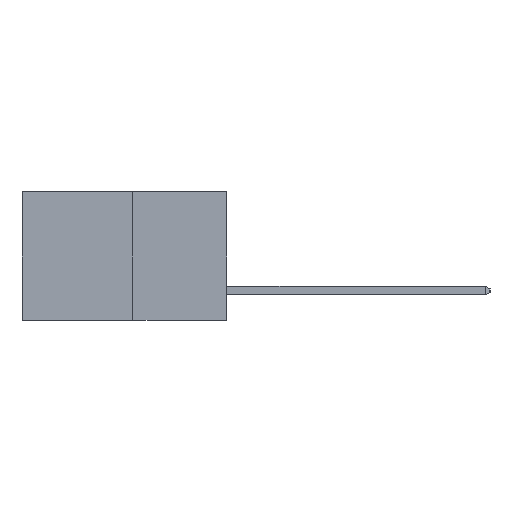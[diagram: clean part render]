
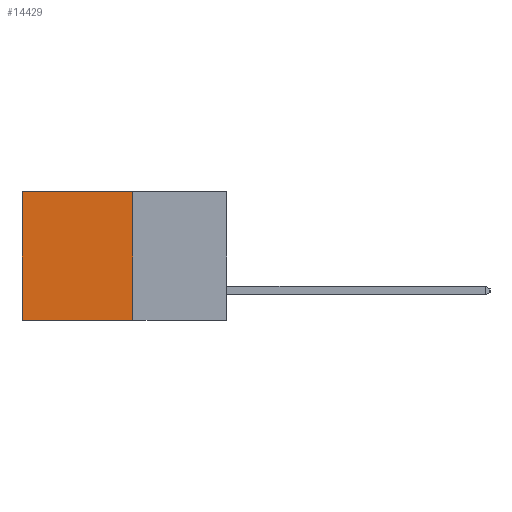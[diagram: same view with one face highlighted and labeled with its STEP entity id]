
A CAD part, left-side view. The second image highlights one B-rep face of the part: STEP entity #14429.
In plain terms, the highlighted planar face has unit normal (-1, 0, 0).
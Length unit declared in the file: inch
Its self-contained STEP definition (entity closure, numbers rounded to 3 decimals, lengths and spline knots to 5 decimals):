
#193 = CARTESIAN_POINT ( 'NONE',  ( 0.277, 0.27, -0.37 ) ) ;
#195 = CARTESIAN_POINT ( 'NONE',  ( 0.277, 0.59, -0.37 ) ) ;
#869 = VECTOR ( 'NONE', #995, 39.37008 ) ;
#995 = DIRECTION ( 'NONE',  ( 0., 0., -1. ) ) ;
#1195 = EDGE_LOOP ( 'NONE', ( #20347, #8211, #4440, #3607 ) ) ;
#1644 = CARTESIAN_POINT ( 'NONE',  ( 0.277, 0.27, -0.37 ) ) ;
#3379 = LINE ( 'NONE', #17132, #8006 ) ;
#3607 = ORIENTED_EDGE ( 'NONE', *, *, #5370, .T. ) ;
#3786 = DIRECTION ( 'NONE',  ( 1., 0., 0. ) ) ;
#4333 = VERTEX_POINT ( 'NONE', #16127 ) ;
#4440 = ORIENTED_EDGE ( 'NONE', *, *, #21651, .F. ) ;
#5370 = EDGE_CURVE ( 'NONE', #9644, #12560, #3379, .T. ) ;
#5723 = EDGE_CURVE ( 'NONE', #12560, #4333, #15222, .T. ) ;
#5804 = DIRECTION ( 'NONE',  ( 0., 0., -1. ) ) ;
#5979 = LINE ( 'NONE', #16025, #10527 ) ;
#6331 = LINE ( 'NONE', #20558, #10337 ) ;
#8006 = VECTOR ( 'NONE', #17205, 39.37008 ) ;
#8211 = ORIENTED_EDGE ( 'NONE', *, *, #9606, .F. ) ;
#9606 = EDGE_CURVE ( 'NONE', #20811, #4333, #6331, .T. ) ;
#9644 = VERTEX_POINT ( 'NONE', #19019 ) ;
#10337 = VECTOR ( 'NONE', #12186, 39.37008 ) ;
#10527 = VECTOR ( 'NONE', #5804, 39.37008 ) ;
#12186 = DIRECTION ( 'NONE',  ( 0., 1., 0. ) ) ;
#12560 = VERTEX_POINT ( 'NONE', #12705 ) ;
#12705 = CARTESIAN_POINT ( 'NONE',  ( 0.277, 0.59, 0. ) ) ;
#13376 = FACE_OUTER_BOUND ( 'NONE', #1195, .T. ) ;
#14107 = PLANE ( 'NONE',  #21374 ) ;
#14429 = ADVANCED_FACE ( 'NONE', ( #13376 ), #14107, .F. ) ;
#15222 = LINE ( 'NONE', #195, #869 ) ;
#15788 = DIRECTION ( 'NONE',  ( 0., 0., -1. ) ) ;
#16025 = CARTESIAN_POINT ( 'NONE',  ( 0.277, 0.27, -0.37 ) ) ;
#16127 = CARTESIAN_POINT ( 'NONE',  ( 0.277, 0.59, -0.37 ) ) ;
#17132 = CARTESIAN_POINT ( 'NONE',  ( 0.277, 0.27, 0. ) ) ;
#17205 = DIRECTION ( 'NONE',  ( 0., 1., 0. ) ) ;
#19019 = CARTESIAN_POINT ( 'NONE',  ( 0.277, 0.27, 0. ) ) ;
#20347 = ORIENTED_EDGE ( 'NONE', *, *, #5723, .T. ) ;
#20558 = CARTESIAN_POINT ( 'NONE',  ( 0.277, 0.27, -0.37 ) ) ;
#20811 = VERTEX_POINT ( 'NONE', #1644 ) ;
#21374 = AXIS2_PLACEMENT_3D ( 'NONE', #193, #3786, #15788 ) ;
#21651 = EDGE_CURVE ( 'NONE', #9644, #20811, #5979, .T. ) ;
